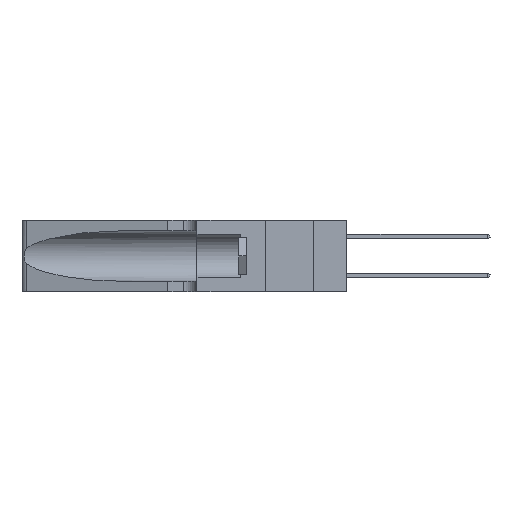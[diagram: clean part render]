
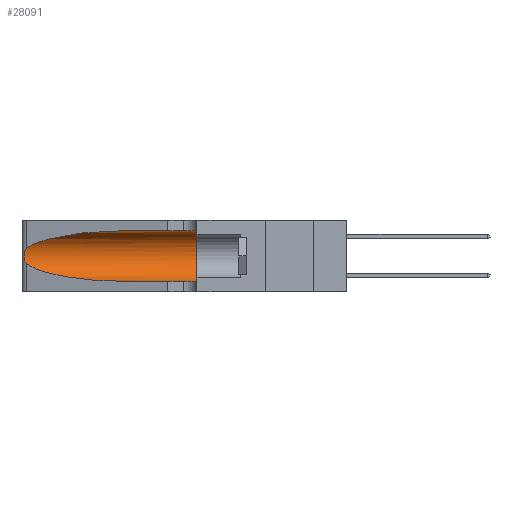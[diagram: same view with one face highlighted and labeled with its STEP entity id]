
A CAD part, left-side view. The second image highlights one B-rep face of the part: STEP entity #28091.
In plain terms, the highlighted cylindrical face has radius 3.308 mm (diameter 6.617 mm), a partial arc.
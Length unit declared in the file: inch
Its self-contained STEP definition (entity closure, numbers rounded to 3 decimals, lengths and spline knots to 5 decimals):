
#1005 = CARTESIAN_POINT ( 'NONE',  ( 0.25555, 1.22993, 0.14849 ) ) ;
#2779 = CARTESIAN_POINT ( 'NONE',  ( 0.18966, 0.96281, 0.05475 ) ) ;
#3812 = ORIENTED_EDGE ( 'NONE', *, *, #13810, .F. ) ;
#4371 = CARTESIAN_POINT ( 'NONE',  ( 0.1305, 0.35, 0.185 ) ) ;
#4736 = CARTESIAN_POINT ( 'NONE',  ( 0.25487, 1.22718, 0.22369 ) ) ;
#5936 = EDGE_CURVE ( 'NONE', #41499, #19230, #16321, .T. ) ;
#6616 = EDGE_LOOP ( 'NONE', ( #31313, #24118, #14700, #34946, #27376, #3812 ) ) ;
#6617 = VECTOR ( 'NONE', #7794, 39.37008 ) ;
#7569 = DIRECTION ( 'NONE',  ( 0., -1., 0. ) ) ;
#7794 = DIRECTION ( 'NONE',  ( 0., -1., 0. ) ) ;
#8363 = DIRECTION ( 'NONE',  ( 0., 0., 1. ) ) ;
#8720 = CARTESIAN_POINT ( 'NONE',  ( 0.25787, 1.23484, 0.2124 ) ) ;
#8734 = CYLINDRICAL_SURFACE ( 'NONE', #39281, 0.13025 ) ;
#12654 = CARTESIAN_POINT ( 'NONE',  ( 0.26018, 1.23835, 0.19895 ) ) ;
#13030 = DIRECTION ( 'NONE',  ( 0., -1., 0. ) ) ;
#13810 = EDGE_CURVE ( 'NONE', #21546, #29260, #19311, .T. ) ;
#14700 = ORIENTED_EDGE ( 'NONE', *, *, #16298, .T. ) ;
#15333 = CARTESIAN_POINT ( 'NONE',  ( 0.1305, 1.61858, 0.05475 ) ) ;
#16298 = EDGE_CURVE ( 'NONE', #19230, #48488, #48298, .T. ) ;
#16321 = B_SPLINE_CURVE_WITH_KNOTS ( 'NONE', 3,
 ( #4736, #24279, #28144, #8720, #35791, #12654, #39610, #16610, #43436, #20525, #47278, #24443, #1005, #28292 ),
 .UNSPECIFIED., .F., .F.,
 ( 4, 2, 2, 2, 2, 2, 4 ),
 ( 0., 0.00027, 0.00053, 0.00107, 0.0016, 0.00187, 0.00214 ),
 .UNSPECIFIED. ) ;
#16610 = CARTESIAN_POINT ( 'NONE',  ( 0.26075, 1.23896, 0.178 ) ) ;
#18776 = CARTESIAN_POINT ( 'NONE',  ( 0.2373, 1.15595, 0.28018 ) ) ;
#19230 = VERTEX_POINT ( 'NONE', #39036 ) ;
#19311 = LINE ( 'NONE', #36154, #39678 ) ;
#20310 = EDGE_CURVE ( 'NONE', #21546, #41499, #39438, .T. ) ;
#20525 = CARTESIAN_POINT ( 'NONE',  ( 0.25856, 1.23593, 0.16098 ) ) ;
#21546 = VERTEX_POINT ( 'NONE', #25783 ) ;
#22295 = CARTESIAN_POINT ( 'NONE',  ( 0.25487, 1.22718, 0.14631 ) ) ;
#23133 = DIRECTION ( 'NONE',  ( 0., 0., -1. ) ) ;
#24118 = ORIENTED_EDGE ( 'NONE', *, *, #5936, .T. ) ;
#24279 = CARTESIAN_POINT ( 'NONE',  ( 0.25555, 1.22994, 0.2215 ) ) ;
#24443 = CARTESIAN_POINT ( 'NONE',  ( 0.25639, 1.23186, 0.15144 ) ) ;
#25783 = CARTESIAN_POINT ( 'NONE',  ( 0.1305, 0.72297, 0.31525 ) ) ;
#27376 = ORIENTED_EDGE ( 'NONE', *, *, #39624, .F. ) ;
#28091 = ADVANCED_FACE ( 'NONE', ( #49724 ), #8734, .F. ) ;
#28144 = CARTESIAN_POINT ( 'NONE',  ( 0.25639, 1.23184, 0.21858 ) ) ;
#28292 = CARTESIAN_POINT ( 'NONE',  ( 0.25487, 1.22718, 0.14631 ) ) ;
#29260 = VERTEX_POINT ( 'NONE', #41357 ) ;
#30013 = CARTESIAN_POINT ( 'NONE',  ( 0.1305, 0.72297, 0.05475 ) ) ;
#31313 = ORIENTED_EDGE ( 'NONE', *, *, #20310, .T. ) ;
#31582 = DIRECTION ( 'NONE',  ( 0., 1., 0. ) ) ;
#32415 = CIRCLE ( 'NONE', #42297, 0.13025 ) ;
#34946 = ORIENTED_EDGE ( 'NONE', *, *, #42400, .T. ) ;
#34982 = CARTESIAN_POINT ( 'NONE',  ( 0.1305, 0.72297, 0.05475 ) ) ;
#35791 = CARTESIAN_POINT ( 'NONE',  ( 0.25854, 1.2359, 0.20912 ) ) ;
#36154 = CARTESIAN_POINT ( 'NONE',  ( 0.1305, 1.61858, 0.31525 ) ) ;
#37917 = CARTESIAN_POINT ( 'NONE',  ( 0.1305, 0.72297, 0.31525 ) ) ;
#38706 = LINE ( 'NONE', #15333, #6617 ) ;
#39036 = CARTESIAN_POINT ( 'NONE',  ( 0.25487, 1.22718, 0.14631 ) ) ;
#39281 = AXIS2_PLACEMENT_3D ( 'NONE', #49851, #7569, #23133 ) ;
#39438 =( BOUNDED_CURVE ( )  B_SPLINE_CURVE ( 3, ( #37917, #41715, #18776, #45547 ),
 .UNSPECIFIED., .F., .F. ) 
 B_SPLINE_CURVE_WITH_KNOTS ( ( 4, 4 ),
 ( 1.5708, 2.84003 ),
 .UNSPECIFIED. ) 
 CURVE ( )  GEOMETRIC_REPRESENTATION_ITEM ( )  RATIONAL_B_SPLINE_CURVE ( ( 1., 0.87, 0.87, 1. ) ) 
 REPRESENTATION_ITEM ( '' )  );
#39610 = CARTESIAN_POINT ( 'NONE',  ( 0.26075, 1.23896, 0.19203 ) ) ;
#39624 = EDGE_CURVE ( 'NONE', #29260, #48950, #32415, .T. ) ;
#39678 = VECTOR ( 'NONE', #13030, 39.37008 ) ;
#41357 = CARTESIAN_POINT ( 'NONE',  ( 0.1305, 0.35, 0.31525 ) ) ;
#41499 = VERTEX_POINT ( 'NONE', #46280 ) ;
#41715 = CARTESIAN_POINT ( 'NONE',  ( 0.18966, 0.96281, 0.31525 ) ) ;
#42297 = AXIS2_PLACEMENT_3D ( 'NONE', #4371, #31582, #8363 ) ;
#42400 = EDGE_CURVE ( 'NONE', #48488, #48950, #38706, .T. ) ;
#43436 = CARTESIAN_POINT ( 'NONE',  ( 0.26017, 1.23833, 0.17102 ) ) ;
#45547 = CARTESIAN_POINT ( 'NONE',  ( 0.25487, 1.22718, 0.22369 ) ) ;
#46280 = CARTESIAN_POINT ( 'NONE',  ( 0.25487, 1.22718, 0.22369 ) ) ;
#47278 = CARTESIAN_POINT ( 'NONE',  ( 0.25789, 1.23486, 0.15765 ) ) ;
#48298 =( BOUNDED_CURVE ( )  B_SPLINE_CURVE ( 3, ( #22295, #49054, #2779, #30013 ),
 .UNSPECIFIED., .F., .F. ) 
 B_SPLINE_CURVE_WITH_KNOTS ( ( 4, 4 ),
 ( 3.44316, 4.71239 ),
 .UNSPECIFIED. ) 
 CURVE ( )  GEOMETRIC_REPRESENTATION_ITEM ( )  RATIONAL_B_SPLINE_CURVE ( ( 1., 0.87, 0.87, 1. ) ) 
 REPRESENTATION_ITEM ( '' )  );
#48488 = VERTEX_POINT ( 'NONE', #34982 ) ;
#48943 = CARTESIAN_POINT ( 'NONE',  ( 0.1305, 0.35, 0.05475 ) ) ;
#48950 = VERTEX_POINT ( 'NONE', #48943 ) ;
#49054 = CARTESIAN_POINT ( 'NONE',  ( 0.2373, 1.15595, 0.08982 ) ) ;
#49724 = FACE_OUTER_BOUND ( 'NONE', #6616, .T. ) ;
#49851 = CARTESIAN_POINT ( 'NONE',  ( 0.1305, 1.61858, 0.185 ) ) ;
